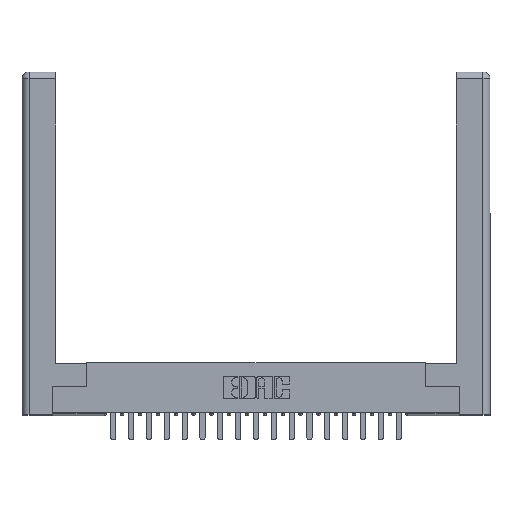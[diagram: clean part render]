
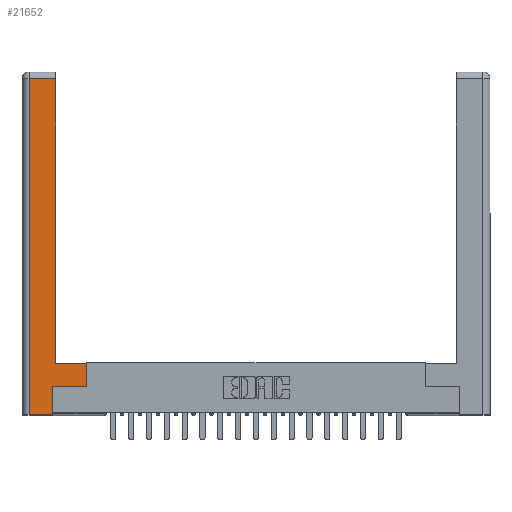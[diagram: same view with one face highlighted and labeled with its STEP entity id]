
A CAD part, top view. The second image highlights one B-rep face of the part: STEP entity #21652.
In plain terms, the highlighted planar face has unit normal (0, 0, 1).
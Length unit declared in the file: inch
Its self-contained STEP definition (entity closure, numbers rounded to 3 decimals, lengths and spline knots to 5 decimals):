
#60 = DIRECTION ( 'NONE',  ( -1., 0., 0. ) ) ;
#464 = ORIENTED_EDGE ( 'NONE', *, *, #17028, .T. ) ;
#672 = DIRECTION ( 'NONE',  ( 1., 0., 0. ) ) ;
#776 = PLANE ( 'NONE',  #21055 ) ;
#1659 = VERTEX_POINT ( 'NONE', #13329 ) ;
#2578 = CARTESIAN_POINT ( 'NONE',  ( 0.265, 0., 0. ) ) ;
#2889 = VECTOR ( 'NONE', #17568, 39.37008 ) ;
#3616 = VERTEX_POINT ( 'NONE', #18083 ) ;
#3847 = EDGE_CURVE ( 'NONE', #16593, #3616, #12620, .T. ) ;
#3878 = VECTOR ( 'NONE', #23852, 39.37008 ) ;
#4318 = CARTESIAN_POINT ( 'NONE',  ( 0.265, 0., 0. ) ) ;
#4384 = EDGE_CURVE ( 'NONE', #11841, #6980, #20413, .T. ) ;
#4498 = CARTESIAN_POINT ( 'NONE',  ( 0.265, 0.245, 0. ) ) ;
#4623 = LINE ( 'NONE', #4498, #2889 ) ;
#4748 = EDGE_CURVE ( 'NONE', #10504, #11841, #10521, .T. ) ;
#4848 = EDGE_LOOP ( 'NONE', ( #12917, #23222, #16950, #17503, #464, #6959, #21415, #23460 ) ) ;
#5261 = DIRECTION ( 'NONE',  ( -1., 0., 0. ) ) ;
#5597 = CARTESIAN_POINT ( 'NONE',  ( 0.565, 0.245, 0. ) ) ;
#5640 = CARTESIAN_POINT ( 'NONE',  ( 0.295, 2.94, 0. ) ) ;
#6850 = CARTESIAN_POINT ( 'NONE',  ( 0.0615, 2.94, 0. ) ) ;
#6959 = ORIENTED_EDGE ( 'NONE', *, *, #3847, .T. ) ;
#6980 = VERTEX_POINT ( 'NONE', #2578 ) ;
#7163 = LINE ( 'NONE', #12622, #9210 ) ;
#7442 = DIRECTION ( 'NONE',  ( 1., 0., 0. ) ) ;
#7994 = EDGE_CURVE ( 'NONE', #3616, #20617, #7163, .T. ) ;
#8149 = EDGE_CURVE ( 'NONE', #20617, #1659, #17907, .T. ) ;
#9060 = EDGE_CURVE ( 'NONE', #23467, #10504, #11735, .T. ) ;
#9210 = VECTOR ( 'NONE', #23934, 39.37008 ) ;
#9648 = DIRECTION ( 'NONE',  ( 0., 1., 0. ) ) ;
#9948 = VECTOR ( 'NONE', #672, 39.37008 ) ;
#9985 = CARTESIAN_POINT ( 'NONE',  ( 0.565, 0.45, 0. ) ) ;
#10504 = VERTEX_POINT ( 'NONE', #6850 ) ;
#10521 = LINE ( 'NONE', #20173, #3878 ) ;
#10569 = VECTOR ( 'NONE', #5261, 39.37008 ) ;
#11139 = CARTESIAN_POINT ( 'NONE',  ( 0.295, 0.45, 0. ) ) ;
#11735 = LINE ( 'NONE', #16371, #10569 ) ;
#11841 = VERTEX_POINT ( 'NONE', #14539 ) ;
#12166 = CARTESIAN_POINT ( 'NONE',  ( 0.265, 0.245, 0. ) ) ;
#12369 = VECTOR ( 'NONE', #60, 39.37008 ) ;
#12620 = LINE ( 'NONE', #5597, #20175 ) ;
#12622 = CARTESIAN_POINT ( 'NONE',  ( 0.565, 0.45, 0. ) ) ;
#12917 = ORIENTED_EDGE ( 'NONE', *, *, #21487, .T. ) ;
#13329 = CARTESIAN_POINT ( 'NONE',  ( 0.295, 0.45, 0. ) ) ;
#14539 = CARTESIAN_POINT ( 'NONE',  ( 0.0615, 0., 0. ) ) ;
#14831 = LINE ( 'NONE', #15103, #19196 ) ;
#15103 = CARTESIAN_POINT ( 'NONE',  ( 0.295, 3., 0. ) ) ;
#15699 = DIRECTION ( 'NONE',  ( -1., 0., 0. ) ) ;
#15724 = FACE_OUTER_BOUND ( 'NONE', #4848, .T. ) ;
#16371 = CARTESIAN_POINT ( 'NONE',  ( 0.0615, 2.94, 0. ) ) ;
#16593 = VERTEX_POINT ( 'NONE', #12166 ) ;
#16950 = ORIENTED_EDGE ( 'NONE', *, *, #4748, .T. ) ;
#17028 = EDGE_CURVE ( 'NONE', #6980, #16593, #4623, .T. ) ;
#17305 = DIRECTION ( 'NONE',  ( 0., 0., -1. ) ) ;
#17503 = ORIENTED_EDGE ( 'NONE', *, *, #4384, .T. ) ;
#17568 = DIRECTION ( 'NONE',  ( 0., 1., 0. ) ) ;
#17907 = LINE ( 'NONE', #11139, #12369 ) ;
#18083 = CARTESIAN_POINT ( 'NONE',  ( 0.565, 0.245, 0. ) ) ;
#19173 = CARTESIAN_POINT ( 'NONE',  ( 0., 0., 0. ) ) ;
#19196 = VECTOR ( 'NONE', #9648, 39.37008 ) ;
#20173 = CARTESIAN_POINT ( 'NONE',  ( 0.0615, 0., 0. ) ) ;
#20175 = VECTOR ( 'NONE', #7442, 39.37008 ) ;
#20413 = LINE ( 'NONE', #4318, #9948 ) ;
#20617 = VERTEX_POINT ( 'NONE', #9985 ) ;
#21055 = AXIS2_PLACEMENT_3D ( 'NONE', #19173, #17305, #15699 ) ;
#21415 = ORIENTED_EDGE ( 'NONE', *, *, #7994, .T. ) ;
#21487 = EDGE_CURVE ( 'NONE', #1659, #23467, #14831, .T. ) ;
#21652 = ADVANCED_FACE ( 'NONE', ( #15724 ), #776, .F. ) ;
#23222 = ORIENTED_EDGE ( 'NONE', *, *, #9060, .T. ) ;
#23460 = ORIENTED_EDGE ( 'NONE', *, *, #8149, .T. ) ;
#23467 = VERTEX_POINT ( 'NONE', #5640 ) ;
#23852 = DIRECTION ( 'NONE',  ( 0., -1., 0. ) ) ;
#23934 = DIRECTION ( 'NONE',  ( 0., 1., 0. ) ) ;
